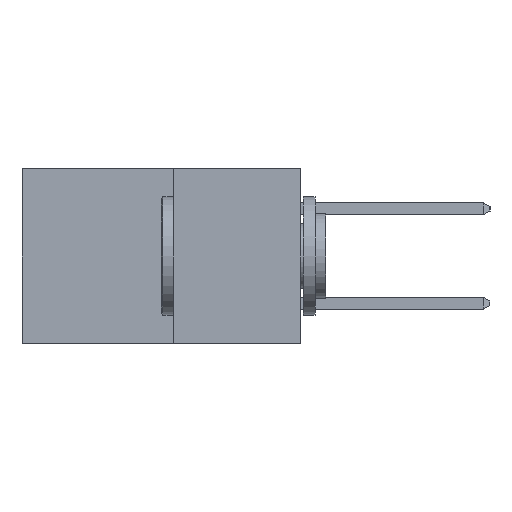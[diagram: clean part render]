
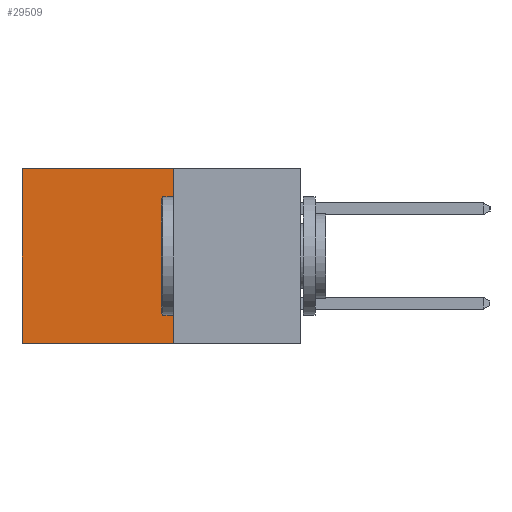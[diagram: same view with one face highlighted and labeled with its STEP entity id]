
A CAD part, left-side view. The second image highlights one B-rep face of the part: STEP entity #29509.
In plain terms, the highlighted planar face has unit normal (-1, 0, 0).
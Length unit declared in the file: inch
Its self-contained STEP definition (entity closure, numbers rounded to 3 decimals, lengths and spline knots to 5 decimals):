
#1518 = AXIS2_PLACEMENT_3D ( 'NONE', #25130, #10682, #28064 ) ;
#2129 = LINE ( 'NONE', #13463, #21286 ) ;
#2364 = EDGE_CURVE ( 'NONE', #9546, #11925, #27751, .T. ) ;
#5715 = LINE ( 'NONE', #20860, #24771 ) ;
#6814 = EDGE_CURVE ( 'NONE', #11925, #22846, #2129, .T. ) ;
#7574 = ORIENTED_EDGE ( 'NONE', *, *, #2364, .F. ) ;
#7727 = PLANE ( 'NONE',  #1518 ) ;
#9401 = FACE_OUTER_BOUND ( 'NONE', #28341, .T. ) ;
#9546 = VERTEX_POINT ( 'NONE', #9706 ) ;
#9706 = CARTESIAN_POINT ( 'NONE',  ( 0.277, 0.27, 0. ) ) ;
#9973 = VECTOR ( 'NONE', #27189, 39.37008 ) ;
#10682 = DIRECTION ( 'NONE',  ( 1., 0., 0. ) ) ;
#11925 = VERTEX_POINT ( 'NONE', #25128 ) ;
#12221 = ORIENTED_EDGE ( 'NONE', *, *, #6814, .F. ) ;
#13035 = ORIENTED_EDGE ( 'NONE', *, *, #18869, .T. ) ;
#13463 = CARTESIAN_POINT ( 'NONE',  ( 0.277, 0.27, -0.37 ) ) ;
#13580 = DIRECTION ( 'NONE',  ( 0., 1., 0. ) ) ;
#14969 = ORIENTED_EDGE ( 'NONE', *, *, #25907, .T. ) ;
#15339 = CARTESIAN_POINT ( 'NONE',  ( 0.277, 0.27, -0.37 ) ) ;
#18869 = EDGE_CURVE ( 'NONE', #9546, #30262, #23196, .T. ) ;
#19724 = CARTESIAN_POINT ( 'NONE',  ( 0.277, 0.27, 0. ) ) ;
#20608 = DIRECTION ( 'NONE',  ( 0., 0., -1. ) ) ;
#20860 = CARTESIAN_POINT ( 'NONE',  ( 0.277, 0.59, -0.37 ) ) ;
#21286 = VECTOR ( 'NONE', #13580, 39.37008 ) ;
#22772 = CARTESIAN_POINT ( 'NONE',  ( 0.277, 0.59, 0. ) ) ;
#22846 = VERTEX_POINT ( 'NONE', #27993 ) ;
#23196 = LINE ( 'NONE', #19724, #9973 ) ;
#24771 = VECTOR ( 'NONE', #30786, 39.37008 ) ;
#25128 = CARTESIAN_POINT ( 'NONE',  ( 0.277, 0.27, -0.37 ) ) ;
#25130 = CARTESIAN_POINT ( 'NONE',  ( 0.277, 0.27, -0.37 ) ) ;
#25907 = EDGE_CURVE ( 'NONE', #30262, #22846, #5715, .T. ) ;
#26961 = VECTOR ( 'NONE', #20608, 39.37008 ) ;
#27189 = DIRECTION ( 'NONE',  ( 0., 1., 0. ) ) ;
#27751 = LINE ( 'NONE', #15339, #26961 ) ;
#27993 = CARTESIAN_POINT ( 'NONE',  ( 0.277, 0.59, -0.37 ) ) ;
#28064 = DIRECTION ( 'NONE',  ( 0., 0., -1. ) ) ;
#28341 = EDGE_LOOP ( 'NONE', ( #14969, #12221, #7574, #13035 ) ) ;
#29509 = ADVANCED_FACE ( 'NONE', ( #9401 ), #7727, .F. ) ;
#30262 = VERTEX_POINT ( 'NONE', #22772 ) ;
#30786 = DIRECTION ( 'NONE',  ( 0., 0., -1. ) ) ;
